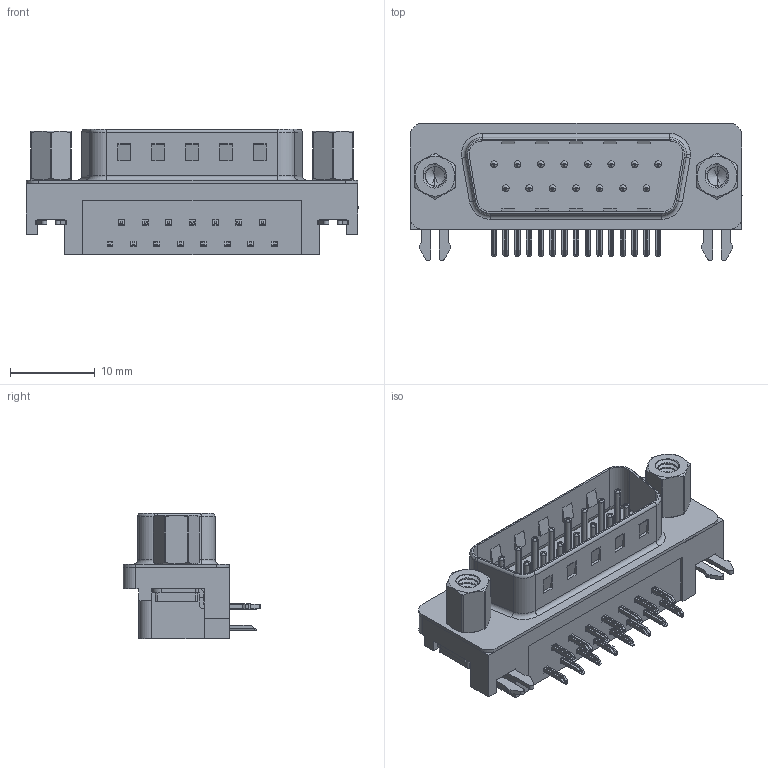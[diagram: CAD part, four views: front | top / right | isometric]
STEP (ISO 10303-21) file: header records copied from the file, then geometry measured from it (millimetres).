
FILE_DESCRIPTION (( 'STEP AP203' ), '1' );
FILE_NAME ('623-015-261-033.STEP', '2018-11-06T12:17:31', ( '' ), ( '' ), 'SwSTEP 2.0', 'SolidWorks 2016', '' );
FILE_SCHEMA (( 'CONFIG_CONTROL_DESIGN' ));
Length unit declared in the file: millimetre
Products named in the file (8): 623 2 Prong Board Lock; 623 4-40 Threaded Rivet; 623 4-40 Hex Standoff 5; 623-015-261-033; 623 Housing_15 Socket; 623 Shell_15 Socket; 623 Contact Bottom; 623 Contact Top
Assembly tree (23 placements, depth 2):
  623-015-261-033
    623 Housing_15 Socket
    623 Shell_15 Socket
    623 Contact Bottom  x7
    623 Contact Top  x8
    623 2 Prong Board Lock  x2
    623 4-40 Threaded Rivet  x2
    623 4-40 Hex Standoff 5  x2
Bounding box: 39.22 x 16.25 x 14.8 mm (x, y, z)
Volume: 3535.7 mm3; surface area: 5417.1 mm2
Topology: 23 solids, 23 shells, 1623 faces, 4073 edges, 2537 vertices
Faces by surface type: plane 943, cylinder 507, torus 121, cone 34, bspline 18
Entity records: 23746 total; most frequent: CARTESIAN_POINT 7772, ORIENTED_EDGE 3064, DIRECTION 3054, EDGE_CURVE 1532, AXIS2_PLACEMENT_3D 1031, VECTOR 992, LINE 992, VERTEX_POINT 981
